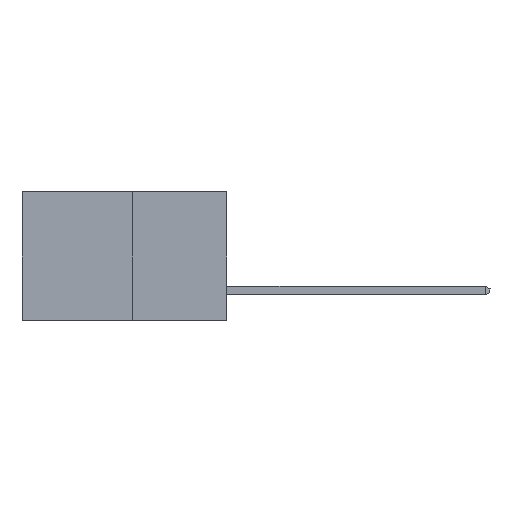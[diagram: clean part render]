
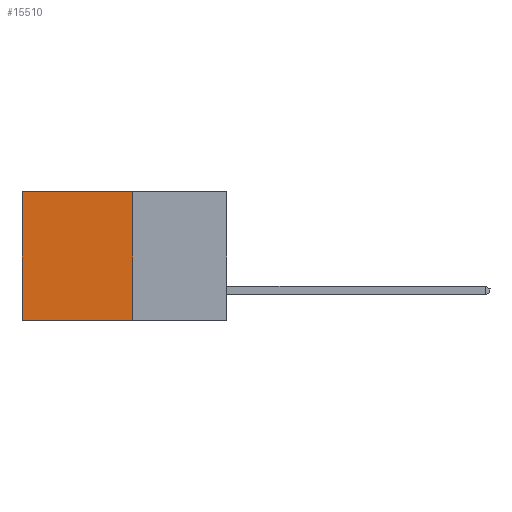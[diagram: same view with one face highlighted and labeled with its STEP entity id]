
A CAD part, left-side view. The second image highlights one B-rep face of the part: STEP entity #15510.
In plain terms, the highlighted planar face has unit normal (-1, 0, 0).
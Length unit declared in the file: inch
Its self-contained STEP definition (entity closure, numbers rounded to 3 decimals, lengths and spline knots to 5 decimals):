
#246 = VERTEX_POINT ( 'NONE', #2720 ) ;
#418 = CARTESIAN_POINT ( 'NONE',  ( 0.277, 0.27, -0.37 ) ) ;
#459 = CARTESIAN_POINT ( 'NONE',  ( 0.277, 0.27, 0. ) ) ;
#470 = VERTEX_POINT ( 'NONE', #1038 ) ;
#1038 = CARTESIAN_POINT ( 'NONE',  ( 0.277, 0.59, 0. ) ) ;
#2099 = EDGE_CURVE ( 'NONE', #470, #246, #2686, .T. ) ;
#2144 = CARTESIAN_POINT ( 'NONE',  ( 0.277, 0.27, 0. ) ) ;
#2404 = EDGE_CURVE ( 'NONE', #3911, #13493, #7395, .T. ) ;
#2686 = LINE ( 'NONE', #10367, #9293 ) ;
#2720 = CARTESIAN_POINT ( 'NONE',  ( 0.277, 0.59, -0.37 ) ) ;
#3227 = VECTOR ( 'NONE', #6049, 39.37008 ) ;
#3694 = EDGE_LOOP ( 'NONE', ( #15306, #5239, #15116, #6950 ) ) ;
#3911 = VERTEX_POINT ( 'NONE', #459 ) ;
#4848 = PLANE ( 'NONE',  #16083 ) ;
#5239 = ORIENTED_EDGE ( 'NONE', *, *, #8625, .F. ) ;
#6049 = DIRECTION ( 'NONE',  ( 0., 1., 0. ) ) ;
#6187 = DIRECTION ( 'NONE',  ( 0., 0., -1. ) ) ;
#6950 = ORIENTED_EDGE ( 'NONE', *, *, #14081, .T. ) ;
#7139 = LINE ( 'NONE', #2144, #3227 ) ;
#7395 = LINE ( 'NONE', #11644, #16867 ) ;
#7689 = DIRECTION ( 'NONE',  ( 0., 0., -1. ) ) ;
#8625 = EDGE_CURVE ( 'NONE', #13493, #246, #8664, .T. ) ;
#8664 = LINE ( 'NONE', #418, #12144 ) ;
#9293 = VECTOR ( 'NONE', #7689, 39.37008 ) ;
#9720 = DIRECTION ( 'NONE',  ( 0., 1., 0. ) ) ;
#10132 = CARTESIAN_POINT ( 'NONE',  ( 0.277, 0.27, -0.37 ) ) ;
#10367 = CARTESIAN_POINT ( 'NONE',  ( 0.277, 0.59, -0.37 ) ) ;
#11644 = CARTESIAN_POINT ( 'NONE',  ( 0.277, 0.27, -0.37 ) ) ;
#11876 = DIRECTION ( 'NONE',  ( 0., 0., -1. ) ) ;
#12144 = VECTOR ( 'NONE', #9720, 39.37008 ) ;
#13493 = VERTEX_POINT ( 'NONE', #13919 ) ;
#13919 = CARTESIAN_POINT ( 'NONE',  ( 0.277, 0.27, -0.37 ) ) ;
#14034 = DIRECTION ( 'NONE',  ( 1., 0., 0. ) ) ;
#14057 = FACE_OUTER_BOUND ( 'NONE', #3694, .T. ) ;
#14081 = EDGE_CURVE ( 'NONE', #3911, #470, #7139, .T. ) ;
#15116 = ORIENTED_EDGE ( 'NONE', *, *, #2404, .F. ) ;
#15306 = ORIENTED_EDGE ( 'NONE', *, *, #2099, .T. ) ;
#15510 = ADVANCED_FACE ( 'NONE', ( #14057 ), #4848, .F. ) ;
#16083 = AXIS2_PLACEMENT_3D ( 'NONE', #10132, #14034, #6187 ) ;
#16867 = VECTOR ( 'NONE', #11876, 39.37008 ) ;
